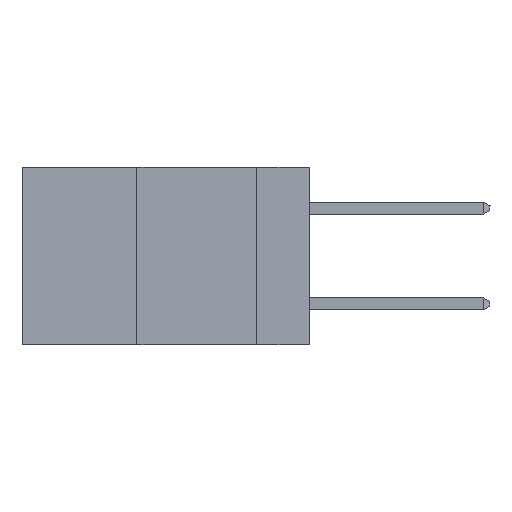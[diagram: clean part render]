
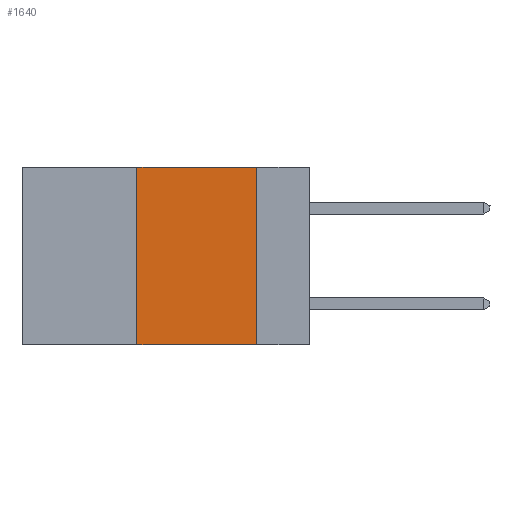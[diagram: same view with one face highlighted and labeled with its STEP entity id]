
A CAD part, left-side view. The second image highlights one B-rep face of the part: STEP entity #1640.
In plain terms, the highlighted planar face has unit normal (-1, 0, 0).
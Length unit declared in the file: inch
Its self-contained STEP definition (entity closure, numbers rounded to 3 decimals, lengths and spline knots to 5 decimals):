
#25 = VECTOR ( 'NONE', #17413, 39.37008 ) ;
#665 = LINE ( 'NONE', #23787, #25 ) ;
#804 = CARTESIAN_POINT ( 'NONE',  ( 0., 0.11, -0.37 ) ) ;
#1041 = CARTESIAN_POINT ( 'NONE',  ( 0., 0.36, -0.37 ) ) ;
#1137 = VERTEX_POINT ( 'NONE', #15864 ) ;
#1275 = EDGE_CURVE ( 'NONE', #20482, #5916, #665, .T. ) ;
#1551 = CARTESIAN_POINT ( 'NONE',  ( 0., 0.36, 0. ) ) ;
#1640 = ADVANCED_FACE ( 'NONE', ( #22217 ), #11794, .F. ) ;
#1996 = ORIENTED_EDGE ( 'NONE', *, *, #16257, .F. ) ;
#3783 = LINE ( 'NONE', #17698, #8999 ) ;
#5521 = LINE ( 'NONE', #5927, #16279 ) ;
#5916 = VERTEX_POINT ( 'NONE', #804 ) ;
#5927 = CARTESIAN_POINT ( 'NONE',  ( 0., 0.6, -0.37 ) ) ;
#6436 = CARTESIAN_POINT ( 'NONE',  ( 0., 0.11, 0. ) ) ;
#7410 = ORIENTED_EDGE ( 'NONE', *, *, #1275, .F. ) ;
#8999 = VECTOR ( 'NONE', #23317, 39.37008 ) ;
#9032 = EDGE_LOOP ( 'NONE', ( #7410, #1996, #11405, #24140 ) ) ;
#9507 = DIRECTION ( 'NONE',  ( 1., 0., 0. ) ) ;
#10970 = DIRECTION ( 'NONE',  ( 0., 0., -1. ) ) ;
#10981 = LINE ( 'NONE', #1551, #15392 ) ;
#11405 = ORIENTED_EDGE ( 'NONE', *, *, #24446, .F. ) ;
#11794 = PLANE ( 'NONE',  #24076 ) ;
#13185 = DIRECTION ( 'NONE',  ( 0., 0., 1. ) ) ;
#15392 = VECTOR ( 'NONE', #13185, 39.37008 ) ;
#15599 = CARTESIAN_POINT ( 'NONE',  ( 0., 0.6, 0. ) ) ;
#15864 = CARTESIAN_POINT ( 'NONE',  ( 0., 0.36, 0. ) ) ;
#16257 = EDGE_CURVE ( 'NONE', #1137, #20482, #3783, .T. ) ;
#16279 = VECTOR ( 'NONE', #19187, 39.37008 ) ;
#17413 = DIRECTION ( 'NONE',  ( 0., 0., -1. ) ) ;
#17698 = CARTESIAN_POINT ( 'NONE',  ( 0., 0.6, 0. ) ) ;
#19010 = EDGE_CURVE ( 'NONE', #24266, #5916, #5521, .T. ) ;
#19187 = DIRECTION ( 'NONE',  ( 0., -1., 0. ) ) ;
#20482 = VERTEX_POINT ( 'NONE', #6436 ) ;
#22217 = FACE_OUTER_BOUND ( 'NONE', #9032, .T. ) ;
#23317 = DIRECTION ( 'NONE',  ( 0., -1., 0. ) ) ;
#23787 = CARTESIAN_POINT ( 'NONE',  ( 0., 0.11, 0. ) ) ;
#24076 = AXIS2_PLACEMENT_3D ( 'NONE', #15599, #9507, #10970 ) ;
#24140 = ORIENTED_EDGE ( 'NONE', *, *, #19010, .T. ) ;
#24266 = VERTEX_POINT ( 'NONE', #1041 ) ;
#24446 = EDGE_CURVE ( 'NONE', #24266, #1137, #10981, .T. ) ;
